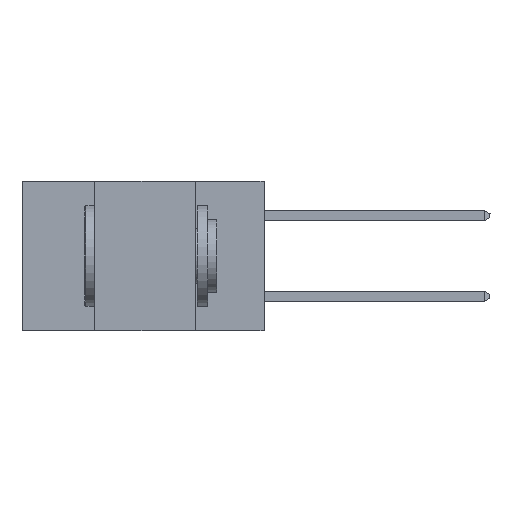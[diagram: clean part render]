
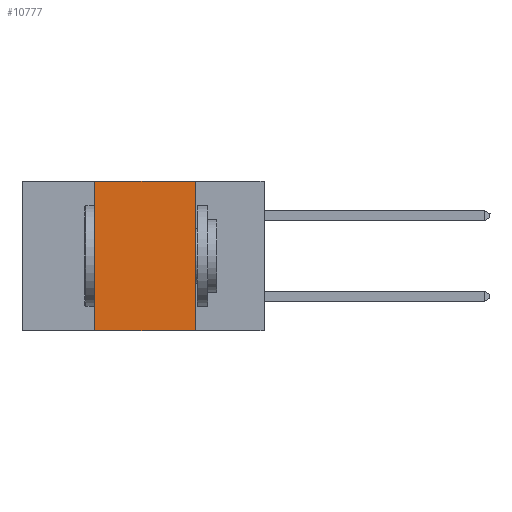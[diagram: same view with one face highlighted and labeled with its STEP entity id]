
A CAD part, left-side view. The second image highlights one B-rep face of the part: STEP entity #10777.
In plain terms, the highlighted planar face has unit normal (-1, 0, 0).
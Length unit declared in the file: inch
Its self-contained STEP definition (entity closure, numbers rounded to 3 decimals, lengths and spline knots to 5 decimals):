
#218 = ORIENTED_EDGE ( 'NONE', *, *, #17644, .T. ) ;
#611 = CARTESIAN_POINT ( 'NONE',  ( 0., 0.42, -0.37 ) ) ;
#1028 = EDGE_CURVE ( 'NONE', #6541, #1598, #12069, .T. ) ;
#1598 = VERTEX_POINT ( 'NONE', #5027 ) ;
#2725 = DIRECTION ( 'NONE',  ( 0., -1., 0. ) ) ;
#3055 = ORIENTED_EDGE ( 'NONE', *, *, #14442, .F. ) ;
#4870 = VECTOR ( 'NONE', #25199, 39.37008 ) ;
#5027 = CARTESIAN_POINT ( 'NONE',  ( 0., 0.17, -0.37 ) ) ;
#5184 = DIRECTION ( 'NONE',  ( 0., 0., 1. ) ) ;
#6247 = PLANE ( 'NONE',  #12374 ) ;
#6541 = VERTEX_POINT ( 'NONE', #11546 ) ;
#8397 = DIRECTION ( 'NONE',  ( 1., 0., 0. ) ) ;
#10723 = ORIENTED_EDGE ( 'NONE', *, *, #18677, .F. ) ;
#10777 = ADVANCED_FACE ( 'NONE', ( #23891 ), #6247, .F. ) ;
#11546 = CARTESIAN_POINT ( 'NONE',  ( 0., 0.17, 0. ) ) ;
#12069 = LINE ( 'NONE', #24657, #22579 ) ;
#12222 = LINE ( 'NONE', #15792, #18520 ) ;
#12374 = AXIS2_PLACEMENT_3D ( 'NONE', #18967, #8397, #23128 ) ;
#12687 = CARTESIAN_POINT ( 'NONE',  ( 0., 0.6, 0. ) ) ;
#13384 = CARTESIAN_POINT ( 'NONE',  ( 0., 0.6, -0.37 ) ) ;
#14442 = EDGE_CURVE ( 'NONE', #16487, #14580, #12222, .T. ) ;
#14580 = VERTEX_POINT ( 'NONE', #20377 ) ;
#15521 = EDGE_LOOP ( 'NONE', ( #16064, #10723, #3055, #218 ) ) ;
#15792 = CARTESIAN_POINT ( 'NONE',  ( 0., 0.42, -0.37 ) ) ;
#16064 = ORIENTED_EDGE ( 'NONE', *, *, #1028, .F. ) ;
#16487 = VERTEX_POINT ( 'NONE', #611 ) ;
#17644 = EDGE_CURVE ( 'NONE', #16487, #1598, #18242, .T. ) ;
#18242 = LINE ( 'NONE', #13384, #18881 ) ;
#18520 = VECTOR ( 'NONE', #5184, 39.37008 ) ;
#18677 = EDGE_CURVE ( 'NONE', #14580, #6541, #21454, .T. ) ;
#18881 = VECTOR ( 'NONE', #2725, 39.37008 ) ;
#18967 = CARTESIAN_POINT ( 'NONE',  ( 0., 0.6, 0. ) ) ;
#20377 = CARTESIAN_POINT ( 'NONE',  ( 0., 0.42, 0. ) ) ;
#21454 = LINE ( 'NONE', #12687, #4870 ) ;
#21557 = DIRECTION ( 'NONE',  ( 0., 0., -1. ) ) ;
#22579 = VECTOR ( 'NONE', #21557, 39.37008 ) ;
#23128 = DIRECTION ( 'NONE',  ( 0., 0., -1. ) ) ;
#23891 = FACE_OUTER_BOUND ( 'NONE', #15521, .T. ) ;
#24657 = CARTESIAN_POINT ( 'NONE',  ( 0., 0.17, -0.37 ) ) ;
#25199 = DIRECTION ( 'NONE',  ( 0., -1., 0. ) ) ;
